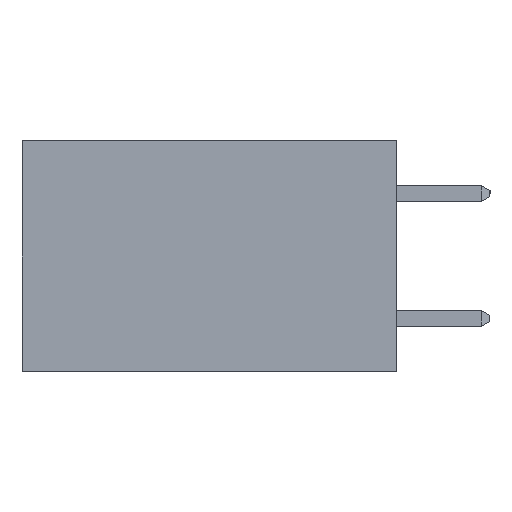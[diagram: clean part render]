
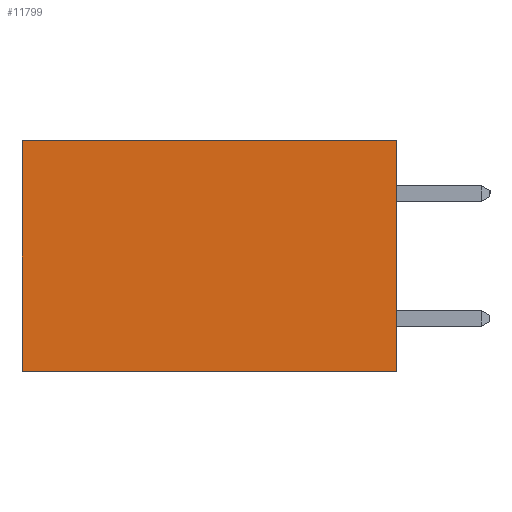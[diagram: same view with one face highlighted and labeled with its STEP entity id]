
A CAD part, left-side view. The second image highlights one B-rep face of the part: STEP entity #11799.
In plain terms, the highlighted planar face has unit normal (-1, 0, 0).
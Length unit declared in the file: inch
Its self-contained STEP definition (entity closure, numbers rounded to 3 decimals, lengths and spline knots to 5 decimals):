
#47 = CARTESIAN_POINT ( 'NONE',  ( 0.2615, 0., 0. ) ) ;
#355 = ORIENTED_EDGE ( 'NONE', *, *, #2285, .T. ) ;
#600 = ORIENTED_EDGE ( 'NONE', *, *, #6777, .T. ) ;
#818 = CARTESIAN_POINT ( 'NONE',  ( 0.2615, 0., -0.37 ) ) ;
#1281 = VERTEX_POINT ( 'NONE', #47 ) ;
#1449 = VERTEX_POINT ( 'NONE', #818 ) ;
#1454 = CARTESIAN_POINT ( 'NONE',  ( 0.2615, 0., 0. ) ) ;
#2285 = EDGE_CURVE ( 'NONE', #11306, #14759, #9961, .T. ) ;
#2843 = EDGE_LOOP ( 'NONE', ( #355, #13785, #15101, #600 ) ) ;
#3664 = LINE ( 'NONE', #5059, #6032 ) ;
#4673 = EDGE_CURVE ( 'NONE', #1281, #1449, #4964, .T. ) ;
#4685 = EDGE_CURVE ( 'NONE', #1449, #14759, #3664, .T. ) ;
#4964 = LINE ( 'NONE', #18739, #15516 ) ;
#5059 = CARTESIAN_POINT ( 'NONE',  ( 0.2615, 0., -0.37 ) ) ;
#5507 = DIRECTION ( 'NONE',  ( 0., 0., -1. ) ) ;
#6032 = VECTOR ( 'NONE', #6654, 39.37008 ) ;
#6071 = FACE_OUTER_BOUND ( 'NONE', #2843, .T. ) ;
#6654 = DIRECTION ( 'NONE',  ( 0., 1., 0. ) ) ;
#6777 = EDGE_CURVE ( 'NONE', #1281, #11306, #8996, .T. ) ;
#7109 = CARTESIAN_POINT ( 'NONE',  ( 0.2615, 0.6, -0.37 ) ) ;
#7559 = DIRECTION ( 'NONE',  ( 0., 0., -1. ) ) ;
#8228 = DIRECTION ( 'NONE',  ( 0., 0., -1. ) ) ;
#8996 = LINE ( 'NONE', #1454, #15526 ) ;
#9766 = DIRECTION ( 'NONE',  ( 0., 1., 0. ) ) ;
#9961 = LINE ( 'NONE', #7109, #15129 ) ;
#11306 = VERTEX_POINT ( 'NONE', #16791 ) ;
#11799 = ADVANCED_FACE ( 'NONE', ( #6071 ), #15374, .F. ) ;
#12207 = CARTESIAN_POINT ( 'NONE',  ( 0.2615, 0., -0.37 ) ) ;
#12302 = DIRECTION ( 'NONE',  ( 1., 0., 0. ) ) ;
#13459 = AXIS2_PLACEMENT_3D ( 'NONE', #12207, #12302, #7559 ) ;
#13785 = ORIENTED_EDGE ( 'NONE', *, *, #4685, .F. ) ;
#14759 = VERTEX_POINT ( 'NONE', #16995 ) ;
#15101 = ORIENTED_EDGE ( 'NONE', *, *, #4673, .F. ) ;
#15129 = VECTOR ( 'NONE', #5507, 39.37008 ) ;
#15374 = PLANE ( 'NONE',  #13459 ) ;
#15516 = VECTOR ( 'NONE', #8228, 39.37008 ) ;
#15526 = VECTOR ( 'NONE', #9766, 39.37008 ) ;
#16791 = CARTESIAN_POINT ( 'NONE',  ( 0.2615, 0.6, 0. ) ) ;
#16995 = CARTESIAN_POINT ( 'NONE',  ( 0.2615, 0.6, -0.37 ) ) ;
#18739 = CARTESIAN_POINT ( 'NONE',  ( 0.2615, 0., -0.37 ) ) ;
